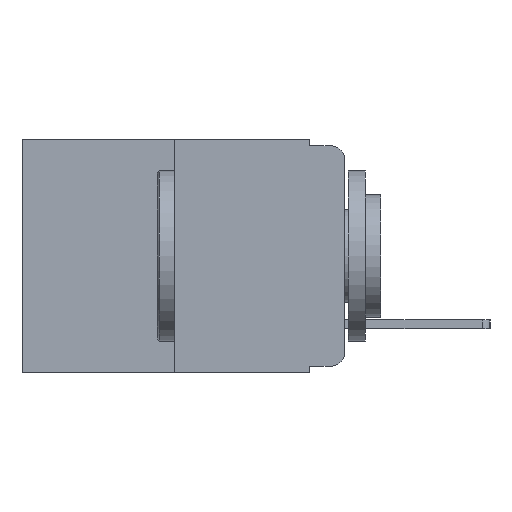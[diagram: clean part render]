
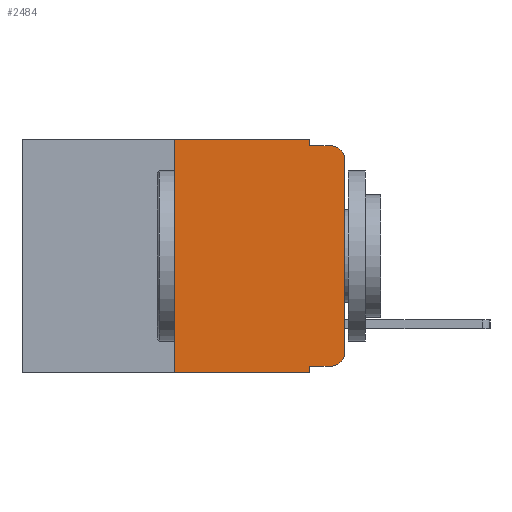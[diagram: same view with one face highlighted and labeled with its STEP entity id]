
A CAD part, left-side view. The second image highlights one B-rep face of the part: STEP entity #2484.
In plain terms, the highlighted planar face has unit normal (-1, 0, 0).
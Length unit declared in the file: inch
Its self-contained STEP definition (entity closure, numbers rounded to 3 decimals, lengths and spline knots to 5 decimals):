
#107 = CARTESIAN_POINT ( 'NONE',  ( 0., 0.25, 0. ) ) ;
#406 = EDGE_CURVE ( 'NONE', #1912, #4757, #10134, .T. ) ;
#566 = CARTESIAN_POINT ( 'NONE',  ( 0., 0.051, 0. ) ) ;
#600 = VERTEX_POINT ( 'NONE', #908 ) ;
#746 = DIRECTION ( 'NONE',  ( 0., 0., -1. ) ) ;
#908 = CARTESIAN_POINT ( 'NONE',  ( 0., 0.02, -0.333 ) ) ;
#972 = VERTEX_POINT ( 'NONE', #10320 ) ;
#1007 = LINE ( 'NONE', #13458, #3731 ) ;
#1560 = VERTEX_POINT ( 'NONE', #3600 ) ;
#1692 = DIRECTION ( 'NONE',  ( 0., -1., 0. ) ) ;
#1694 = EDGE_CURVE ( 'NONE', #1912, #11064, #7432, .T. ) ;
#1696 = VERTEX_POINT ( 'NONE', #9806 ) ;
#1912 = VERTEX_POINT ( 'NONE', #4101 ) ;
#2029 = ORIENTED_EDGE ( 'NONE', *, *, #406, .F. ) ;
#2146 = LINE ( 'NONE', #4331, #7578 ) ;
#2282 = VERTEX_POINT ( 'NONE', #11648 ) ;
#2301 = CARTESIAN_POINT ( 'NONE',  ( 0., 0.473, -0.343 ) ) ;
#2484 = ADVANCED_FACE ( 'NONE', ( #5428 ), #11550, .F. ) ;
#2619 = CARTESIAN_POINT ( 'NONE',  ( 0., 0.051, -0.01 ) ) ;
#2792 = DIRECTION ( 'NONE',  ( 0., 0., 1. ) ) ;
#3041 = EDGE_CURVE ( 'NONE', #2282, #11064, #9008, .T. ) ;
#3267 = CARTESIAN_POINT ( 'NONE',  ( 0., 0.051, 0. ) ) ;
#3306 = CARTESIAN_POINT ( 'NONE',  ( 0., 0.02, -0.03 ) ) ;
#3526 = CARTESIAN_POINT ( 'NONE',  ( 0., 0.02, -0.313 ) ) ;
#3600 = CARTESIAN_POINT ( 'NONE',  ( 0., 0.02, -0.01 ) ) ;
#3628 = EDGE_CURVE ( 'NONE', #4757, #10099, #1007, .T. ) ;
#3731 = VECTOR ( 'NONE', #14130, 39.37008 ) ;
#3767 = ORIENTED_EDGE ( 'NONE', *, *, #12130, .T. ) ;
#4101 = CARTESIAN_POINT ( 'NONE',  ( 0., 0.25, -0.343 ) ) ;
#4135 = DIRECTION ( 'NONE',  ( 0., 0., -1. ) ) ;
#4331 = CARTESIAN_POINT ( 'NONE',  ( 0., 0., 0. ) ) ;
#4688 = DIRECTION ( 'NONE',  ( 0., 0., -1. ) ) ;
#4699 = VECTOR ( 'NONE', #1692, 39.37008 ) ;
#4700 = DIRECTION ( 'NONE',  ( -1., 0., 0. ) ) ;
#4708 = ORIENTED_EDGE ( 'NONE', *, *, #3628, .F. ) ;
#4757 = VERTEX_POINT ( 'NONE', #107 ) ;
#5428 = FACE_OUTER_BOUND ( 'NONE', #13320, .T. ) ;
#5591 = VECTOR ( 'NONE', #746, 39.37008 ) ;
#6004 = ORIENTED_EDGE ( 'NONE', *, *, #13610, .T. ) ;
#6067 = EDGE_CURVE ( 'NONE', #1696, #1560, #12550, .T. ) ;
#6209 = AXIS2_PLACEMENT_3D ( 'NONE', #3306, #4700, #4135 ) ;
#6267 = VECTOR ( 'NONE', #14809, 39.37008 ) ;
#6347 = ORIENTED_EDGE ( 'NONE', *, *, #14815, .T. ) ;
#6940 = CARTESIAN_POINT ( 'NONE',  ( 0., 0.051, -0.333 ) ) ;
#7101 = VECTOR ( 'NONE', #2792, 39.37008 ) ;
#7238 = DIRECTION ( 'NONE',  ( 1., 0., 0. ) ) ;
#7432 = LINE ( 'NONE', #2301, #4699 ) ;
#7578 = VECTOR ( 'NONE', #14574, 39.37008 ) ;
#7975 = ORIENTED_EDGE ( 'NONE', *, *, #3041, .F. ) ;
#8085 = AXIS2_PLACEMENT_3D ( 'NONE', #11154, #7238, #9665 ) ;
#8121 = CARTESIAN_POINT ( 'NONE',  ( 0., 0.051, -0.343 ) ) ;
#8833 = CARTESIAN_POINT ( 'NONE',  ( 0., 0.051, -0.01 ) ) ;
#8946 = VECTOR ( 'NONE', #14785, 39.37008 ) ;
#9008 = LINE ( 'NONE', #566, #5591 ) ;
#9296 = LINE ( 'NONE', #6940, #6267 ) ;
#9567 = ORIENTED_EDGE ( 'NONE', *, *, #6067, .T. ) ;
#9665 = DIRECTION ( 'NONE',  ( 0., 0., -1. ) ) ;
#9806 = CARTESIAN_POINT ( 'NONE',  ( 0., 0., -0.03 ) ) ;
#9953 = DIRECTION ( 'NONE',  ( 0., -1., 0. ) ) ;
#10089 = ORIENTED_EDGE ( 'NONE', *, *, #13170, .F. ) ;
#10099 = VERTEX_POINT ( 'NONE', #3267 ) ;
#10134 = LINE ( 'NONE', #12408, #7101 ) ;
#10320 = CARTESIAN_POINT ( 'NONE',  ( 0., 0., -0.313 ) ) ;
#11064 = VERTEX_POINT ( 'NONE', #8121 ) ;
#11079 = VECTOR ( 'NONE', #9953, 39.37008 ) ;
#11154 = CARTESIAN_POINT ( 'NONE',  ( 0., 0.473, 0. ) ) ;
#11223 = VERTEX_POINT ( 'NONE', #2619 ) ;
#11508 = DIRECTION ( 'NONE',  ( -1., 0., 0. ) ) ;
#11550 = PLANE ( 'NONE',  #8085 ) ;
#11648 = CARTESIAN_POINT ( 'NONE',  ( 0., 0.051, -0.333 ) ) ;
#11653 = ORIENTED_EDGE ( 'NONE', *, *, #1694, .T. ) ;
#11871 = ORIENTED_EDGE ( 'NONE', *, *, #14216, .F. ) ;
#11907 = LINE ( 'NONE', #13666, #8946 ) ;
#12122 = AXIS2_PLACEMENT_3D ( 'NONE', #3526, #11508, #4688 ) ;
#12130 = EDGE_CURVE ( 'NONE', #972, #1696, #2146, .T. ) ;
#12408 = CARTESIAN_POINT ( 'NONE',  ( 0., 0.25, 0. ) ) ;
#12550 = CIRCLE ( 'NONE', #6209, 0.02 ) ;
#13170 = EDGE_CURVE ( 'NONE', #11223, #1560, #14063, .T. ) ;
#13320 = EDGE_LOOP ( 'NONE', ( #3767, #9567, #10089, #11871, #4708, #2029, #11653, #7975, #6347, #6004 ) ) ;
#13458 = CARTESIAN_POINT ( 'NONE',  ( 0., 0.473, 0. ) ) ;
#13610 = EDGE_CURVE ( 'NONE', #600, #972, #14051, .T. ) ;
#13666 = CARTESIAN_POINT ( 'NONE',  ( 0., 0.051, 0. ) ) ;
#14051 = CIRCLE ( 'NONE', #12122, 0.02 ) ;
#14063 = LINE ( 'NONE', #8833, #11079 ) ;
#14130 = DIRECTION ( 'NONE',  ( 0., -1., 0. ) ) ;
#14216 = EDGE_CURVE ( 'NONE', #10099, #11223, #11907, .T. ) ;
#14574 = DIRECTION ( 'NONE',  ( 0., 0., 1. ) ) ;
#14785 = DIRECTION ( 'NONE',  ( 0., 0., -1. ) ) ;
#14809 = DIRECTION ( 'NONE',  ( 0., -1., 0. ) ) ;
#14815 = EDGE_CURVE ( 'NONE', #2282, #600, #9296, .T. ) ;
